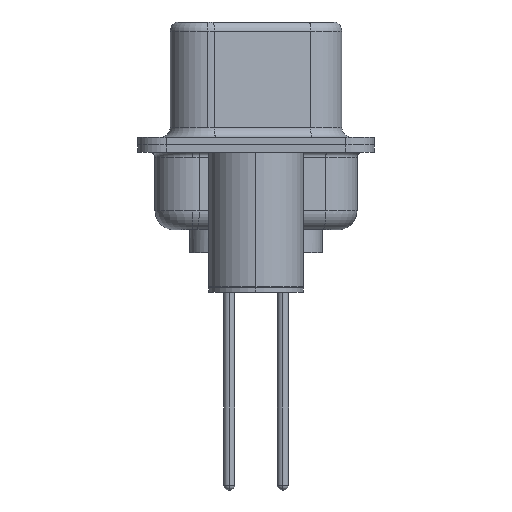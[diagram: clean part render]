
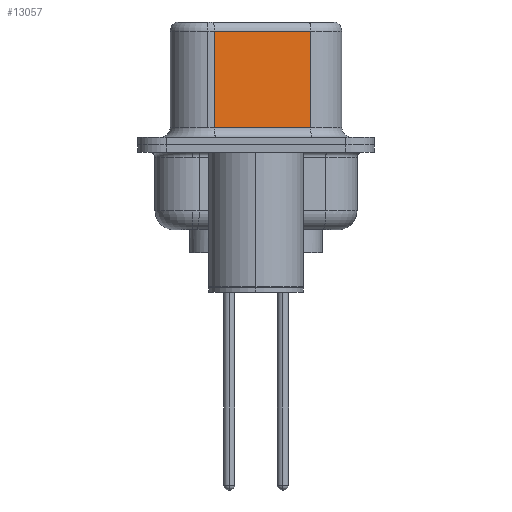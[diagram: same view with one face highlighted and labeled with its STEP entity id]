
A CAD part, left-side view. The second image highlights one B-rep face of the part: STEP entity #13057.
In plain terms, the highlighted planar face has unit normal (-0.985, -0.174, 0).
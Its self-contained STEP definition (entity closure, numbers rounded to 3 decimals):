
#430 = ORIENTED_EDGE ( 'NONE', *, *, #16538, .F. ) ;
#707 = VECTOR ( 'NONE', #7354, 1000. ) ;
#1236 = LINE ( 'NONE', #7677, #12024 ) ;
#2146 = DIRECTION ( 'NONE',  ( 0.985, 0.174, 0. ) ) ;
#2246 = CARTESIAN_POINT ( 'NONE',  ( 4.58, -2.897, 6.52 ) ) ;
#2434 = VERTEX_POINT ( 'NONE', #9210 ) ;
#3454 = CARTESIAN_POINT ( 'NONE',  ( 3.68, 2.203, 6.52 ) ) ;
#4038 = DIRECTION ( 'NONE',  ( -0.174, 0.985, 0. ) ) ;
#4853 = CARTESIAN_POINT ( 'NONE',  ( 4.58, -2.897, 6.02 ) ) ;
#4907 = ORIENTED_EDGE ( 'NONE', *, *, #19501, .T. ) ;
#5658 = CARTESIAN_POINT ( 'NONE',  ( 4.58, -2.897, 6.02 ) ) ;
#6190 = VERTEX_POINT ( 'NONE', #17717 ) ;
#7354 = DIRECTION ( 'NONE',  ( 0.174, -0.985, 0. ) ) ;
#7677 = CARTESIAN_POINT ( 'NONE',  ( 4.58, -2.897, 6.52 ) ) ;
#8720 = DIRECTION ( 'NONE',  ( -0.174, 0.985, 0. ) ) ;
#9210 = CARTESIAN_POINT ( 'NONE',  ( 3.68, 2.203, 6.02 ) ) ;
#9707 = VECTOR ( 'NONE', #10041, 1000. ) ;
#10009 = VECTOR ( 'NONE', #4038, 1000. ) ;
#10041 = DIRECTION ( 'NONE',  ( 0., 0., -1. ) ) ;
#10340 = PLANE ( 'NONE',  #19730 ) ;
#10547 = VERTEX_POINT ( 'NONE', #4853 ) ;
#10814 = CARTESIAN_POINT ( 'NONE',  ( 4.58, -2.897, 0.9 ) ) ;
#11978 = FACE_OUTER_BOUND ( 'NONE', #14674, .T. ) ;
#12024 = VECTOR ( 'NONE', #15705, 1000. ) ;
#12595 = CARTESIAN_POINT ( 'NONE',  ( 4.58, -2.897, 0.9 ) ) ;
#13057 = ADVANCED_FACE ( 'NONE', ( #11978 ), #10340, .F. ) ;
#13730 = ORIENTED_EDGE ( 'NONE', *, *, #17821, .T. ) ;
#14674 = EDGE_LOOP ( 'NONE', ( #430, #4907, #19708, #13730 ) ) ;
#15705 = DIRECTION ( 'NONE',  ( 0., 0., -1. ) ) ;
#15841 = LINE ( 'NONE', #10814, #707 ) ;
#16538 = EDGE_CURVE ( 'NONE', #10547, #17766, #1236, .T. ) ;
#16902 = LINE ( 'NONE', #5658, #10009 ) ;
#17717 = CARTESIAN_POINT ( 'NONE',  ( 3.68, 2.203, 0.9 ) ) ;
#17766 = VERTEX_POINT ( 'NONE', #12595 ) ;
#17821 = EDGE_CURVE ( 'NONE', #6190, #17766, #15841, .T. ) ;
#18369 = LINE ( 'NONE', #3454, #9707 ) ;
#19501 = EDGE_CURVE ( 'NONE', #10547, #2434, #16902, .T. ) ;
#19708 = ORIENTED_EDGE ( 'NONE', *, *, #20478, .T. ) ;
#19730 = AXIS2_PLACEMENT_3D ( 'NONE', #2246, #2146, #8720 ) ;
#20478 = EDGE_CURVE ( 'NONE', #2434, #6190, #18369, .T. ) ;
